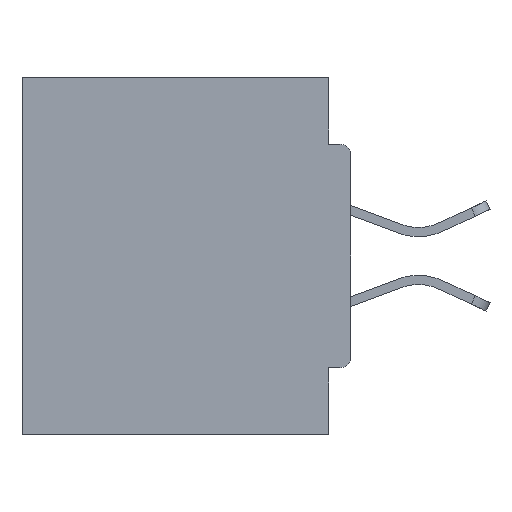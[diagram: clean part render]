
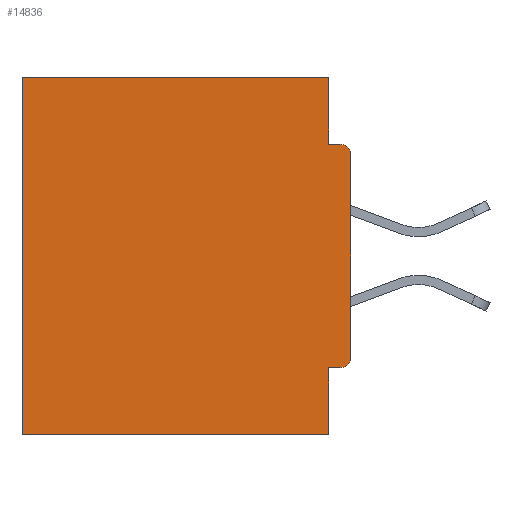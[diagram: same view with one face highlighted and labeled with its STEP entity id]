
A CAD part, left-side view. The second image highlights one B-rep face of the part: STEP entity #14836.
In plain terms, the highlighted planar face has unit normal (-1, 0, 0).
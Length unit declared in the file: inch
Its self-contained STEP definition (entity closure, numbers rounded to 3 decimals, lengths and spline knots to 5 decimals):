
#197 = EDGE_CURVE ( 'NONE', #5788, #43459, #37725, .T. ) ;
#1014 = FACE_OUTER_BOUND ( 'NONE', #28179, .T. ) ;
#1248 = VECTOR ( 'NONE', #39407, 39.37008 ) ;
#2075 = ORIENTED_EDGE ( 'NONE', *, *, #197, .F. ) ;
#5788 = VERTEX_POINT ( 'NONE', #41539 ) ;
#6126 = ORIENTED_EDGE ( 'NONE', *, *, #27631, .F. ) ;
#6465 = LINE ( 'NONE', #16195, #17098 ) ;
#6623 = VERTEX_POINT ( 'NONE', #46344 ) ;
#7032 = DIRECTION ( 'NONE',  ( 0., 0., -1. ) ) ;
#7282 = CARTESIAN_POINT ( 'NONE',  ( 0.298, 0.031, -0.5 ) ) ;
#8104 = EDGE_CURVE ( 'NONE', #5788, #21042, #15434, .T. ) ;
#8432 = ORIENTED_EDGE ( 'NONE', *, *, #43111, .T. ) ;
#8565 = VERTEX_POINT ( 'NONE', #7282 ) ;
#9321 = ORIENTED_EDGE ( 'NONE', *, *, #22263, .F. ) ;
#10006 = LINE ( 'NONE', #20789, #29035 ) ;
#10765 = CARTESIAN_POINT ( 'NONE',  ( 0.298, 0., 0. ) ) ;
#12249 = DIRECTION ( 'NONE',  ( 0., 0., -1. ) ) ;
#12343 = ORIENTED_EDGE ( 'NONE', *, *, #35512, .F. ) ;
#13117 = ORIENTED_EDGE ( 'NONE', *, *, #34752, .T. ) ;
#13818 = EDGE_CURVE ( 'NONE', #45963, #45747, #17935, .T. ) ;
#13897 = ORIENTED_EDGE ( 'NONE', *, *, #8104, .T. ) ;
#14836 = ADVANCED_FACE ( 'NONE', ( #1014 ), #28585, .F. ) ;
#15434 = CIRCLE ( 'NONE', #42032, 0.015 ) ;
#15491 = CARTESIAN_POINT ( 'NONE',  ( 0.298, 0., 0. ) ) ;
#15815 = VECTOR ( 'NONE', #19582, 39.37008 ) ;
#16195 = CARTESIAN_POINT ( 'NONE',  ( 0.298, 0., 0. ) ) ;
#17098 = VECTOR ( 'NONE', #30734, 39.37008 ) ;
#17145 = ORIENTED_EDGE ( 'NONE', *, *, #23396, .F. ) ;
#17935 = LINE ( 'NONE', #23649, #42041 ) ;
#18129 = DIRECTION ( 'NONE',  ( 1., 0., 0. ) ) ;
#18631 = VERTEX_POINT ( 'NONE', #29299 ) ;
#18811 = EDGE_CURVE ( 'NONE', #33855, #44254, #34816, .T. ) ;
#18975 = DIRECTION ( 'NONE',  ( 0., 0., -1. ) ) ;
#19582 = DIRECTION ( 'NONE',  ( 0., -1., 0. ) ) ;
#20789 = CARTESIAN_POINT ( 'NONE',  ( 0.298, 0., -0.5 ) ) ;
#21042 = VERTEX_POINT ( 'NONE', #43312 ) ;
#21253 = CARTESIAN_POINT ( 'NONE',  ( 0.298, 0.46, 0. ) ) ;
#22263 = EDGE_CURVE ( 'NONE', #18631, #33855, #43772, .T. ) ;
#22682 = DIRECTION ( 'NONE',  ( 0., 0., -1. ) ) ;
#23396 = EDGE_CURVE ( 'NONE', #8565, #45747, #10006, .T. ) ;
#23649 = CARTESIAN_POINT ( 'NONE',  ( 0.298, 0.46, 0. ) ) ;
#24158 = VECTOR ( 'NONE', #7032, 39.37008 ) ;
#24198 = LINE ( 'NONE', #10765, #1248 ) ;
#25801 = DIRECTION ( 'NONE',  ( 0., 1., 0. ) ) ;
#27631 = EDGE_CURVE ( 'NONE', #43459, #8565, #28173, .T. ) ;
#27807 = CARTESIAN_POINT ( 'NONE',  ( 0.298, 0.031, -0.0935 ) ) ;
#28173 = LINE ( 'NONE', #29494, #45597 ) ;
#28179 = EDGE_LOOP ( 'NONE', ( #13117, #30844, #9321, #8432, #40681, #17145, #6126, #2075, #13897, #12343 ) ) ;
#28585 = PLANE ( 'NONE',  #44035 ) ;
#28922 = DIRECTION ( 'NONE',  ( -1., 0., 0. ) ) ;
#29035 = VECTOR ( 'NONE', #38649, 39.37008 ) ;
#29254 = CARTESIAN_POINT ( 'NONE',  ( 0.298, 0.031, -0.4065 ) ) ;
#29299 = CARTESIAN_POINT ( 'NONE',  ( 0.298, 0.031, 0. ) ) ;
#29494 = CARTESIAN_POINT ( 'NONE',  ( 0.298, 0.031, -0.5 ) ) ;
#30734 = DIRECTION ( 'NONE',  ( 0., 1., 0. ) ) ;
#30844 = ORIENTED_EDGE ( 'NONE', *, *, #18811, .F. ) ;
#32015 = AXIS2_PLACEMENT_3D ( 'NONE', #35982, #28922, #36607 ) ;
#33396 = DIRECTION ( 'NONE',  ( 0., 0., -1. ) ) ;
#33855 = VERTEX_POINT ( 'NONE', #27807 ) ;
#34752 = EDGE_CURVE ( 'NONE', #6623, #44254, #37185, .T. ) ;
#34816 = LINE ( 'NONE', #40568, #15815 ) ;
#34845 = CARTESIAN_POINT ( 'NONE',  ( 0.298, 0.46, -0.5 ) ) ;
#35512 = EDGE_CURVE ( 'NONE', #6623, #21042, #24198, .T. ) ;
#35791 = CARTESIAN_POINT ( 'NONE',  ( 0.298, 0., -0.4065 ) ) ;
#35982 = CARTESIAN_POINT ( 'NONE',  ( 0.298, 0.015, -0.1085 ) ) ;
#36607 = DIRECTION ( 'NONE',  ( 0., 0., -1. ) ) ;
#37185 = CIRCLE ( 'NONE', #32015, 0.015 ) ;
#37725 = LINE ( 'NONE', #35791, #39982 ) ;
#38649 = DIRECTION ( 'NONE',  ( 0., 1., 0. ) ) ;
#39407 = DIRECTION ( 'NONE',  ( 0., 0., -1. ) ) ;
#39982 = VECTOR ( 'NONE', #25801, 39.37008 ) ;
#40568 = CARTESIAN_POINT ( 'NONE',  ( 0.298, 0., -0.0935 ) ) ;
#40589 = CARTESIAN_POINT ( 'NONE',  ( 0.298, 0.015, -0.3915 ) ) ;
#40681 = ORIENTED_EDGE ( 'NONE', *, *, #13818, .T. ) ;
#40888 = DIRECTION ( 'NONE',  ( -1., 0., 0. ) ) ;
#41539 = CARTESIAN_POINT ( 'NONE',  ( 0.298, 0.015, -0.4065 ) ) ;
#42000 = CARTESIAN_POINT ( 'NONE',  ( 0.298, 0.015, -0.0935 ) ) ;
#42032 = AXIS2_PLACEMENT_3D ( 'NONE', #40589, #40888, #18975 ) ;
#42041 = VECTOR ( 'NONE', #12249, 39.37008 ) ;
#42910 = CARTESIAN_POINT ( 'NONE',  ( 0.298, 0.031, -0.5 ) ) ;
#43111 = EDGE_CURVE ( 'NONE', #18631, #45963, #6465, .T. ) ;
#43312 = CARTESIAN_POINT ( 'NONE',  ( 0.298, 0., -0.3915 ) ) ;
#43459 = VERTEX_POINT ( 'NONE', #29254 ) ;
#43772 = LINE ( 'NONE', #42910, #24158 ) ;
#44035 = AXIS2_PLACEMENT_3D ( 'NONE', #15491, #18129, #22682 ) ;
#44254 = VERTEX_POINT ( 'NONE', #42000 ) ;
#45597 = VECTOR ( 'NONE', #33396, 39.37008 ) ;
#45747 = VERTEX_POINT ( 'NONE', #34845 ) ;
#45963 = VERTEX_POINT ( 'NONE', #21253 ) ;
#46344 = CARTESIAN_POINT ( 'NONE',  ( 0.298, 0., -0.1085 ) ) ;
